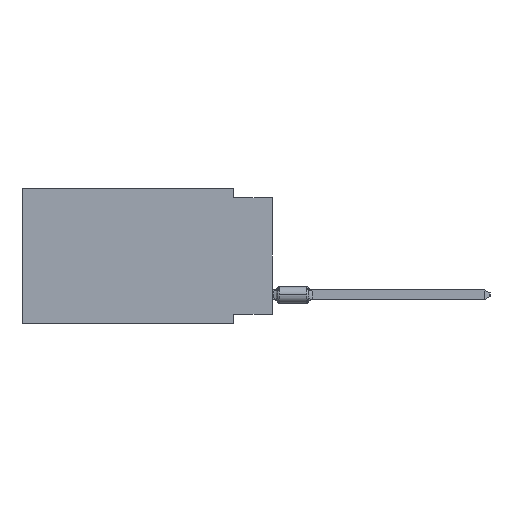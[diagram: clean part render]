
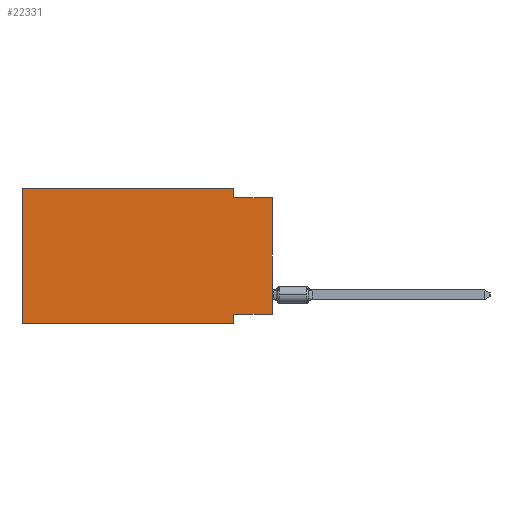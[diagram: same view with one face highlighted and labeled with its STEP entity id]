
A CAD part, left-side view. The second image highlights one B-rep face of the part: STEP entity #22331.
In plain terms, the highlighted planar face has unit normal (-1, 0, 0).
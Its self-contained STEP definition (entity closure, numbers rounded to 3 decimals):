
#36 = LINE ( 'NONE', #20693, #26234 ) ;
#42 = AXIS2_PLACEMENT_3D ( 'NONE', #18832, #4927, #28708 ) ;
#218 = DIRECTION ( 'NONE',  ( 0., 0., 1. ) ) ;
#2035 = ORIENTED_EDGE ( 'NONE', *, *, #20207, .F. ) ;
#4927 = DIRECTION ( 'NONE',  ( 1., 0., 0. ) ) ;
#5222 = VECTOR ( 'NONE', #6634, 1000. ) ;
#6205 = LINE ( 'NONE', #33820, #5222 ) ;
#6634 = DIRECTION ( 'NONE',  ( 0., -1., 0. ) ) ;
#7019 = CARTESIAN_POINT ( 'NONE',  ( 0., 0., -0.635 ) ) ;
#7084 = DIRECTION ( 'NONE',  ( 0., 0., -1. ) ) ;
#7868 = CARTESIAN_POINT ( 'NONE',  ( 0., 2.54, -8.255 ) ) ;
#7964 = VECTOR ( 'NONE', #42703, 1000. ) ;
#10941 = VECTOR ( 'NONE', #7084, 1000. ) ;
#11660 = ORIENTED_EDGE ( 'NONE', *, *, #26126, .T. ) ;
#12268 = ORIENTED_EDGE ( 'NONE', *, *, #31579, .T. ) ;
#13581 = ORIENTED_EDGE ( 'NONE', *, *, #26353, .F. ) ;
#13590 = VERTEX_POINT ( 'NONE', #21230 ) ;
#13813 = EDGE_CURVE ( 'NONE', #34961, #36608, #37956, .T. ) ;
#13823 = CARTESIAN_POINT ( 'NONE',  ( 0., 2.54, -8.89 ) ) ;
#14182 = ORIENTED_EDGE ( 'NONE', *, *, #42199, .F. ) ;
#14289 = CARTESIAN_POINT ( 'NONE',  ( 0., 2.54, 0. ) ) ;
#14714 = LINE ( 'NONE', #13823, #10941 ) ;
#15631 = VERTEX_POINT ( 'NONE', #7868 ) ;
#16686 = ORIENTED_EDGE ( 'NONE', *, *, #37059, .F. ) ;
#18067 = CARTESIAN_POINT ( 'NONE',  ( 0., 16.383, 0. ) ) ;
#18832 = CARTESIAN_POINT ( 'NONE',  ( 0., 16.383, 0. ) ) ;
#20207 = EDGE_CURVE ( 'NONE', #36608, #28346, #30822, .T. ) ;
#20693 = CARTESIAN_POINT ( 'NONE',  ( 0., 0., -8.255 ) ) ;
#21230 = CARTESIAN_POINT ( 'NONE',  ( 0., 0., -8.255 ) ) ;
#21979 = PLANE ( 'NONE',  #42 ) ;
#22331 = ADVANCED_FACE ( 'NONE', ( #32973 ), #21979, .F. ) ;
#22946 = EDGE_CURVE ( 'NONE', #43371, #34961, #33261, .T. ) ;
#23499 = CARTESIAN_POINT ( 'NONE',  ( 0., 16.383, -8.89 ) ) ;
#24468 = CARTESIAN_POINT ( 'NONE',  ( 0., 0., 0. ) ) ;
#24564 = CARTESIAN_POINT ( 'NONE',  ( 0., 2.54, -0.635 ) ) ;
#26126 = EDGE_CURVE ( 'NONE', #34840, #33154, #6205, .T. ) ;
#26131 = CARTESIAN_POINT ( 'NONE',  ( 0., 16.383, 0. ) ) ;
#26234 = VECTOR ( 'NONE', #35510, 1000. ) ;
#26353 = EDGE_CURVE ( 'NONE', #15631, #33154, #14714, .T. ) ;
#26989 = CARTESIAN_POINT ( 'NONE',  ( 0., 0., -0.635 ) ) ;
#28346 = VERTEX_POINT ( 'NONE', #26989 ) ;
#28708 = DIRECTION ( 'NONE',  ( 0., 0., -1. ) ) ;
#29004 = CARTESIAN_POINT ( 'NONE',  ( 0., 16.383, 0. ) ) ;
#29443 = VECTOR ( 'NONE', #218, 1000. ) ;
#30822 = LINE ( 'NONE', #7019, #42240 ) ;
#31241 = CARTESIAN_POINT ( 'NONE',  ( 0., 2.54, 0. ) ) ;
#31579 = EDGE_CURVE ( 'NONE', #13590, #28346, #34812, .T. ) ;
#32871 = LINE ( 'NONE', #26131, #42585 ) ;
#32973 = FACE_OUTER_BOUND ( 'NONE', #39595, .T. ) ;
#33154 = VERTEX_POINT ( 'NONE', #34108 ) ;
#33261 = LINE ( 'NONE', #29004, #7964 ) ;
#33820 = CARTESIAN_POINT ( 'NONE',  ( 0., 16.383, -8.89 ) ) ;
#34108 = CARTESIAN_POINT ( 'NONE',  ( 0., 2.54, -8.89 ) ) ;
#34812 = LINE ( 'NONE', #24468, #29443 ) ;
#34840 = VERTEX_POINT ( 'NONE', #23499 ) ;
#34961 = VERTEX_POINT ( 'NONE', #14289 ) ;
#35510 = DIRECTION ( 'NONE',  ( 0., 1., 0. ) ) ;
#36234 = ORIENTED_EDGE ( 'NONE', *, *, #22946, .F. ) ;
#36608 = VERTEX_POINT ( 'NONE', #24564 ) ;
#37059 = EDGE_CURVE ( 'NONE', #13590, #15631, #36, .T. ) ;
#37784 = DIRECTION ( 'NONE',  ( 0., -1., 0. ) ) ;
#37956 = LINE ( 'NONE', #31241, #41151 ) ;
#38414 = DIRECTION ( 'NONE',  ( 0., 0., -1. ) ) ;
#39595 = EDGE_LOOP ( 'NONE', ( #12268, #2035, #43679, #36234, #14182, #11660, #13581, #16686 ) ) ;
#39832 = DIRECTION ( 'NONE',  ( 0., 0., 1. ) ) ;
#41151 = VECTOR ( 'NONE', #38414, 1000. ) ;
#42199 = EDGE_CURVE ( 'NONE', #34840, #43371, #32871, .T. ) ;
#42240 = VECTOR ( 'NONE', #37784, 1000. ) ;
#42585 = VECTOR ( 'NONE', #39832, 1000. ) ;
#42703 = DIRECTION ( 'NONE',  ( 0., -1., 0. ) ) ;
#43371 = VERTEX_POINT ( 'NONE', #18067 ) ;
#43679 = ORIENTED_EDGE ( 'NONE', *, *, #13813, .F. ) ;
